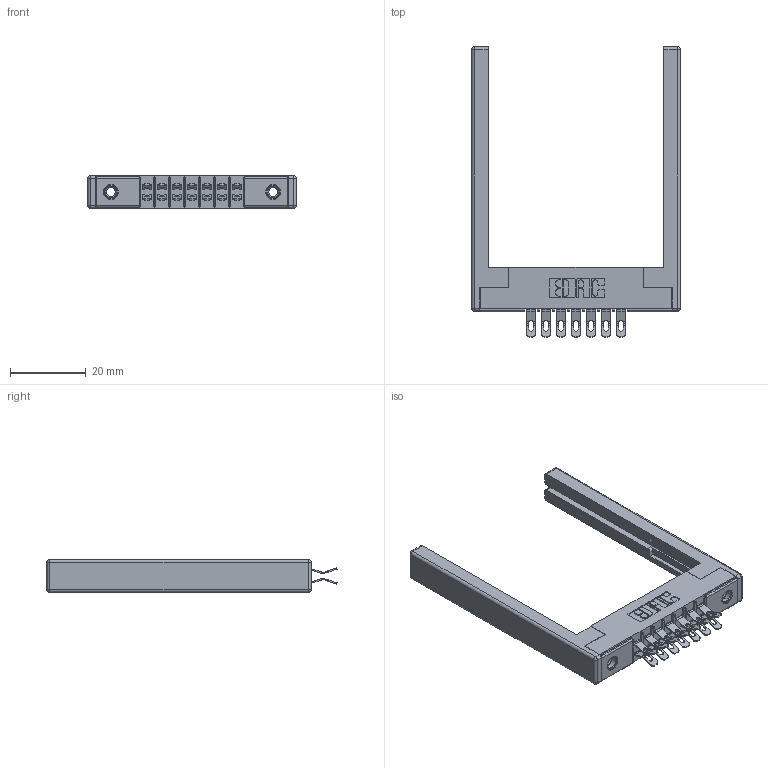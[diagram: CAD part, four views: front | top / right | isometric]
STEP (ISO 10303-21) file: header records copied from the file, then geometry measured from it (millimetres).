
FILE_DESCRIPTION (( 'STEP AP203' ), '1' );
FILE_NAME ('315-014-555-268.STEP', '2019-09-10T13:35:34', ( '' ), ( '' ), 'SwSTEP 2.0', 'SolidWorks 2016', '' );
FILE_SCHEMA (( 'CONFIG_CONTROL_DESIGN' ));
Length unit declared in the file: inch
Products named in the file (5): 305-290-001_555; 305 Part_.156 Dia; 307-220-068; 315-014-555-268; 345-250-001_345-250-001-102
Assembly tree (19 placements, depth 2):
  315-014-555-268
    305 Part_.156 Dia
    305-290-001_555  x14
    345-250-001_345-250-001-102  x2
    307-220-068  x2
Bounding box: 55.17 x 76.71 x 8.71 mm (x, y, z)
Volume: 8101.6 mm3; surface area: 10038.2 mm2
Topology: 19 solids, 19 shells, 1194 faces, 3471 edges, 2254 vertices
Faces by surface type: plane 604, cylinder 538, sphere 36, cone 12, torus 4
Entity records: 15223 total; most frequent: CARTESIAN_POINT 2510, DIRECTION 2470, ORIENTED_EDGE 2468, EDGE_CURVE 1234, VECTOR 930, LINE 930, VERTEX_POINT 794, AXIS2_PLACEMENT_3D 770
